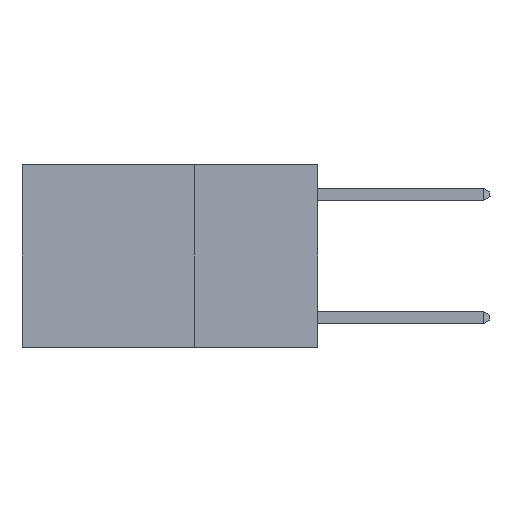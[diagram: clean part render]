
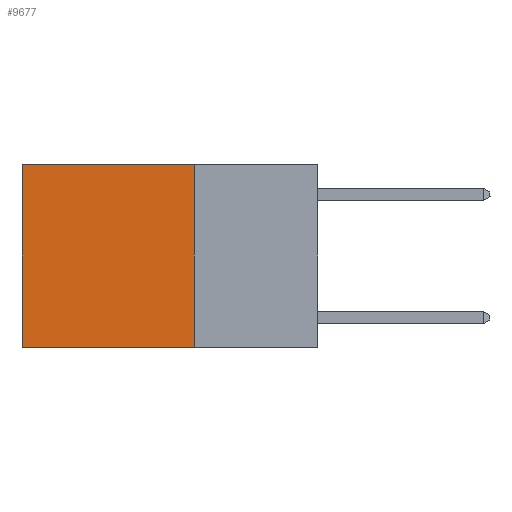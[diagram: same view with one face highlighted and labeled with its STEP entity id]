
A CAD part, left-side view. The second image highlights one B-rep face of the part: STEP entity #9677.
In plain terms, the highlighted planar face has unit normal (-1, 0, 0).
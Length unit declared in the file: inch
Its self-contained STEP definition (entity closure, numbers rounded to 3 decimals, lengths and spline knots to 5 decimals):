
#179 = DIRECTION ( 'NONE',  ( 0., 1., 0. ) ) ;
#508 = CARTESIAN_POINT ( 'NONE',  ( 0.2625, 0.6, 0. ) ) ;
#860 = CARTESIAN_POINT ( 'NONE',  ( 0.2625, 0.25, 0. ) ) ;
#1193 = EDGE_CURVE ( 'NONE', #3012, #6586, #6170, .T. ) ;
#2126 = PLANE ( 'NONE',  #3388 ) ;
#2220 = VECTOR ( 'NONE', #179, 39.37008 ) ;
#2352 = VECTOR ( 'NONE', #6724, 39.37008 ) ;
#2735 = LINE ( 'NONE', #3412, #2352 ) ;
#3012 = VERTEX_POINT ( 'NONE', #9736 ) ;
#3148 = VECTOR ( 'NONE', #3760, 39.37008 ) ;
#3328 = ORIENTED_EDGE ( 'NONE', *, *, #9893, .F. ) ;
#3388 = AXIS2_PLACEMENT_3D ( 'NONE', #10321, #4507, #8530 ) ;
#3412 = CARTESIAN_POINT ( 'NONE',  ( 0.2625, 0.25, 0. ) ) ;
#3760 = DIRECTION ( 'NONE',  ( 0., 0., -1. ) ) ;
#4262 = ORIENTED_EDGE ( 'NONE', *, *, #9166, .F. ) ;
#4497 = EDGE_LOOP ( 'NONE', ( #7662, #4262, #3328, #10209 ) ) ;
#4507 = DIRECTION ( 'NONE',  ( 1., 0., 0. ) ) ;
#4858 = LINE ( 'NONE', #860, #7677 ) ;
#5294 = CARTESIAN_POINT ( 'NONE',  ( 0.2625, 0.25, 0. ) ) ;
#5358 = CARTESIAN_POINT ( 'NONE',  ( 0.2625, 0.6, -0.37 ) ) ;
#6170 = LINE ( 'NONE', #508, #3148 ) ;
#6586 = VERTEX_POINT ( 'NONE', #5358 ) ;
#6724 = DIRECTION ( 'NONE',  ( 0., 1., 0. ) ) ;
#7096 = VERTEX_POINT ( 'NONE', #5294 ) ;
#7537 = CARTESIAN_POINT ( 'NONE',  ( 0.2625, 0.25, -0.37 ) ) ;
#7662 = ORIENTED_EDGE ( 'NONE', *, *, #1193, .T. ) ;
#7677 = VECTOR ( 'NONE', #8089, 39.37008 ) ;
#7750 = EDGE_CURVE ( 'NONE', #7096, #3012, #2735, .T. ) ;
#7845 = FACE_OUTER_BOUND ( 'NONE', #4497, .T. ) ;
#8089 = DIRECTION ( 'NONE',  ( 0., 0., -1. ) ) ;
#8530 = DIRECTION ( 'NONE',  ( 0., 0., -1. ) ) ;
#8827 = CARTESIAN_POINT ( 'NONE',  ( 0.2625, 0.25, -0.37 ) ) ;
#9012 = LINE ( 'NONE', #7537, #2220 ) ;
#9166 = EDGE_CURVE ( 'NONE', #9795, #6586, #9012, .T. ) ;
#9677 = ADVANCED_FACE ( 'NONE', ( #7845 ), #2126, .F. ) ;
#9736 = CARTESIAN_POINT ( 'NONE',  ( 0.2625, 0.6, 0. ) ) ;
#9795 = VERTEX_POINT ( 'NONE', #8827 ) ;
#9893 = EDGE_CURVE ( 'NONE', #7096, #9795, #4858, .T. ) ;
#10209 = ORIENTED_EDGE ( 'NONE', *, *, #7750, .T. ) ;
#10321 = CARTESIAN_POINT ( 'NONE',  ( 0.2625, 0.25, 0. ) ) ;
